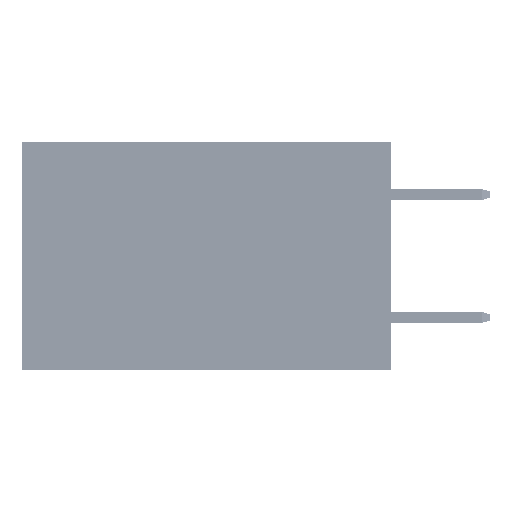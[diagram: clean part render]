
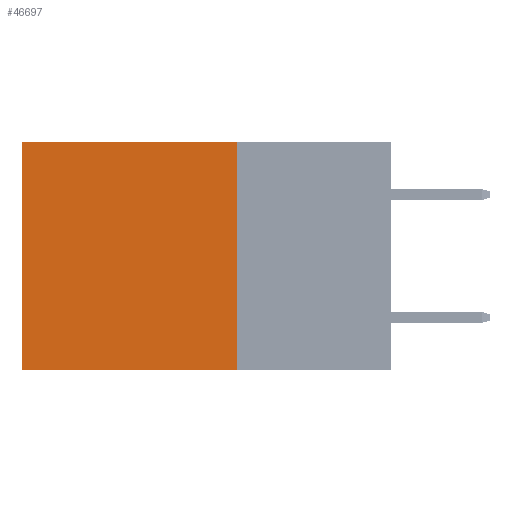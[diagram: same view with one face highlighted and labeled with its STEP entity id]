
A CAD part, left-side view. The second image highlights one B-rep face of the part: STEP entity #46697.
In plain terms, the highlighted planar face has unit normal (-1, 0, 0).
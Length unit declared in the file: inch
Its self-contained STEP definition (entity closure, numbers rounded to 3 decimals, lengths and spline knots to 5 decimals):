
#1127 = EDGE_CURVE ( 'NONE', #47535, #6447, #22647, .T. ) ;
#2957 = EDGE_CURVE ( 'NONE', #15508, #6447, #48634, .T. ) ;
#4488 = AXIS2_PLACEMENT_3D ( 'NONE', #42303, #20865, #29395 ) ;
#4663 = ORIENTED_EDGE ( 'NONE', *, *, #34641, .F. ) ;
#6447 = VERTEX_POINT ( 'NONE', #38407 ) ;
#7394 = VERTEX_POINT ( 'NONE', #51588 ) ;
#10380 = EDGE_CURVE ( 'NONE', #7394, #47535, #53107, .T. ) ;
#13740 = VECTOR ( 'NONE', #39771, 39.37008 ) ;
#15508 = VERTEX_POINT ( 'NONE', #25599 ) ;
#16867 = PLANE ( 'NONE',  #4488 ) ;
#18730 = VECTOR ( 'NONE', #30944, 39.37008 ) ;
#19439 = ORIENTED_EDGE ( 'NONE', *, *, #1127, .T. ) ;
#19520 = DIRECTION ( 'NONE',  ( 0., 1., 0. ) ) ;
#20865 = DIRECTION ( 'NONE',  ( 1., 0., 0. ) ) ;
#21506 = CARTESIAN_POINT ( 'NONE',  ( 0.2875, 0.6, 0. ) ) ;
#22647 = LINE ( 'NONE', #47312, #18730 ) ;
#25599 = CARTESIAN_POINT ( 'NONE',  ( 0.2875, 0.25, -0.37 ) ) ;
#29296 = LINE ( 'NONE', #36299, #13740 ) ;
#29395 = DIRECTION ( 'NONE',  ( 0., 0., -1. ) ) ;
#30944 = DIRECTION ( 'NONE',  ( 0., 0., -1. ) ) ;
#31864 = CARTESIAN_POINT ( 'NONE',  ( 0.2875, 0.25, 0. ) ) ;
#34641 = EDGE_CURVE ( 'NONE', #7394, #15508, #29296, .T. ) ;
#36299 = CARTESIAN_POINT ( 'NONE',  ( 0.2875, 0.25, 0. ) ) ;
#38407 = CARTESIAN_POINT ( 'NONE',  ( 0.2875, 0.6, -0.37 ) ) ;
#39771 = DIRECTION ( 'NONE',  ( 0., 0., -1. ) ) ;
#40420 = ORIENTED_EDGE ( 'NONE', *, *, #2957, .F. ) ;
#40565 = FACE_OUTER_BOUND ( 'NONE', #41332, .T. ) ;
#40709 = CARTESIAN_POINT ( 'NONE',  ( 0.2875, 0.25, -0.37 ) ) ;
#41332 = EDGE_LOOP ( 'NONE', ( #19439, #40420, #4663, #53421 ) ) ;
#42303 = CARTESIAN_POINT ( 'NONE',  ( 0.2875, 0.25, 0. ) ) ;
#44704 = VECTOR ( 'NONE', #49266, 39.37008 ) ;
#46697 = ADVANCED_FACE ( 'NONE', ( #40565 ), #16867, .F. ) ;
#47312 = CARTESIAN_POINT ( 'NONE',  ( 0.2875, 0.6, 0. ) ) ;
#47535 = VERTEX_POINT ( 'NONE', #21506 ) ;
#48634 = LINE ( 'NONE', #40709, #44704 ) ;
#49266 = DIRECTION ( 'NONE',  ( 0., 1., 0. ) ) ;
#51141 = VECTOR ( 'NONE', #19520, 39.37008 ) ;
#51588 = CARTESIAN_POINT ( 'NONE',  ( 0.2875, 0.25, 0. ) ) ;
#53107 = LINE ( 'NONE', #31864, #51141 ) ;
#53421 = ORIENTED_EDGE ( 'NONE', *, *, #10380, .T. ) ;
